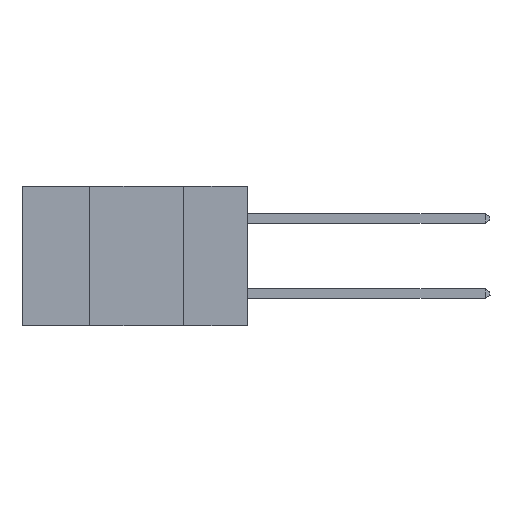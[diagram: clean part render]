
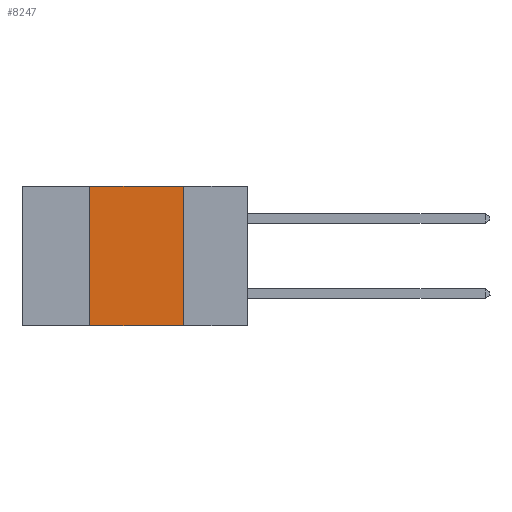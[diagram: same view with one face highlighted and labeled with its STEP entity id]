
A CAD part, left-side view. The second image highlights one B-rep face of the part: STEP entity #8247.
In plain terms, the highlighted planar face has unit normal (-1, 0, 0).
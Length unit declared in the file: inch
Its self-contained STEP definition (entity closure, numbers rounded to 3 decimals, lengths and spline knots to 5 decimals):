
#683 = DIRECTION ( 'NONE',  ( 1., 0., 0. ) ) ;
#834 = DIRECTION ( 'NONE',  ( 0., 0., -1. ) ) ;
#1085 = DIRECTION ( 'NONE',  ( 0., 0., 1. ) ) ;
#1645 = VERTEX_POINT ( 'NONE', #11545 ) ;
#1704 = DIRECTION ( 'NONE',  ( 0., -1., 0. ) ) ;
#1873 = CARTESIAN_POINT ( 'NONE',  ( 0., 0.6, -0.37 ) ) ;
#2927 = EDGE_CURVE ( 'NONE', #14359, #3139, #5827, .T. ) ;
#3139 = VERTEX_POINT ( 'NONE', #16413 ) ;
#3417 = CARTESIAN_POINT ( 'NONE',  ( 0., 0.17, 0. ) ) ;
#4153 = FACE_OUTER_BOUND ( 'NONE', #13303, .T. ) ;
#4694 = DIRECTION ( 'NONE',  ( 0., 0., -1. ) ) ;
#5827 = LINE ( 'NONE', #3417, #9830 ) ;
#5947 = LINE ( 'NONE', #1873, #16575 ) ;
#6226 = CARTESIAN_POINT ( 'NONE',  ( 0., 0.6, 0. ) ) ;
#6891 = ORIENTED_EDGE ( 'NONE', *, *, #12858, .F. ) ;
#7102 = CARTESIAN_POINT ( 'NONE',  ( 0., 0.42, 0. ) ) ;
#7628 = DIRECTION ( 'NONE',  ( 0., -1., 0. ) ) ;
#8247 = ADVANCED_FACE ( 'NONE', ( #4153 ), #16198, .F. ) ;
#8268 = CARTESIAN_POINT ( 'NONE',  ( 0., 0.6, 0. ) ) ;
#8297 = VECTOR ( 'NONE', #1085, 39.37008 ) ;
#9196 = EDGE_CURVE ( 'NONE', #1645, #3139, #5947, .T. ) ;
#9830 = VECTOR ( 'NONE', #4694, 39.37008 ) ;
#10609 = LINE ( 'NONE', #14924, #8297 ) ;
#10705 = LINE ( 'NONE', #6226, #12905 ) ;
#11156 = ORIENTED_EDGE ( 'NONE', *, *, #15534, .F. ) ;
#11225 = AXIS2_PLACEMENT_3D ( 'NONE', #8268, #683, #834 ) ;
#11545 = CARTESIAN_POINT ( 'NONE',  ( 0., 0.42, -0.37 ) ) ;
#12858 = EDGE_CURVE ( 'NONE', #16430, #14359, #10705, .T. ) ;
#12905 = VECTOR ( 'NONE', #7628, 39.37008 ) ;
#12949 = ORIENTED_EDGE ( 'NONE', *, *, #9196, .T. ) ;
#13184 = CARTESIAN_POINT ( 'NONE',  ( 0., 0.17, 0. ) ) ;
#13303 = EDGE_LOOP ( 'NONE', ( #14824, #6891, #11156, #12949 ) ) ;
#14359 = VERTEX_POINT ( 'NONE', #13184 ) ;
#14824 = ORIENTED_EDGE ( 'NONE', *, *, #2927, .F. ) ;
#14924 = CARTESIAN_POINT ( 'NONE',  ( 0., 0.42, 0. ) ) ;
#15534 = EDGE_CURVE ( 'NONE', #1645, #16430, #10609, .T. ) ;
#16198 = PLANE ( 'NONE',  #11225 ) ;
#16413 = CARTESIAN_POINT ( 'NONE',  ( 0., 0.17, -0.37 ) ) ;
#16430 = VERTEX_POINT ( 'NONE', #7102 ) ;
#16575 = VECTOR ( 'NONE', #1704, 39.37008 ) ;
